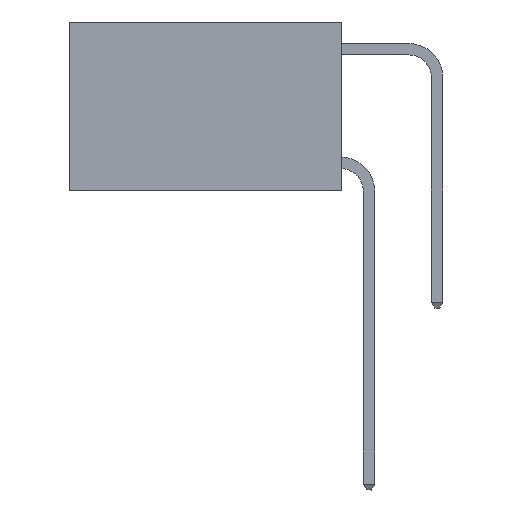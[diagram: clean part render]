
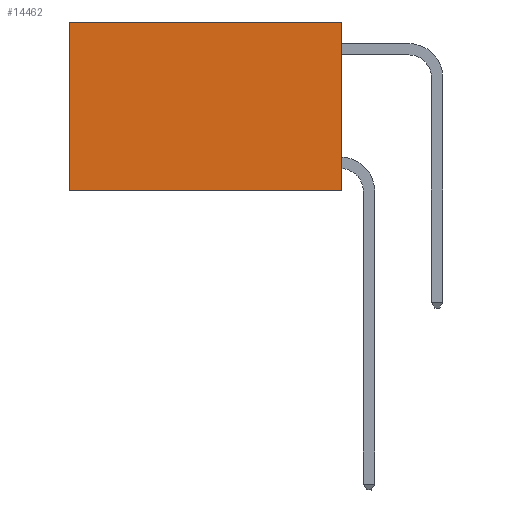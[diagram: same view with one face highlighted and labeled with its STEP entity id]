
A CAD part, left-side view. The second image highlights one B-rep face of the part: STEP entity #14462.
In plain terms, the highlighted planar face has unit normal (-1, 0, 0).
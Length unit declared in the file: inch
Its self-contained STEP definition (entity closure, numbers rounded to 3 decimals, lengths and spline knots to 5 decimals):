
#859 = ORIENTED_EDGE ( 'NONE', *, *, #15998, .F. ) ;
#1146 = LINE ( 'NONE', #4782, #16189 ) ;
#4782 = CARTESIAN_POINT ( 'NONE',  ( 0.2625, 0., 0. ) ) ;
#6386 = VERTEX_POINT ( 'NONE', #22277 ) ;
#6719 = CARTESIAN_POINT ( 'NONE',  ( 0.2625, 0., 0. ) ) ;
#6848 = CARTESIAN_POINT ( 'NONE',  ( 0.2625, 0., -0.37 ) ) ;
#7182 = PLANE ( 'NONE',  #23463 ) ;
#8040 = VECTOR ( 'NONE', #8683, 39.37008 ) ;
#8683 = DIRECTION ( 'NONE',  ( 0., 0., -1. ) ) ;
#8804 = DIRECTION ( 'NONE',  ( 0., 1., 0. ) ) ;
#9157 = DIRECTION ( 'NONE',  ( 0., 0., -1. ) ) ;
#9379 = VECTOR ( 'NONE', #8804, 39.37008 ) ;
#10536 = VECTOR ( 'NONE', #21991, 39.37008 ) ;
#10845 = VERTEX_POINT ( 'NONE', #13858 ) ;
#12106 = FACE_OUTER_BOUND ( 'NONE', #24737, .T. ) ;
#12195 = CARTESIAN_POINT ( 'NONE',  ( 0.2625, 0.6, -0.37 ) ) ;
#13858 = CARTESIAN_POINT ( 'NONE',  ( 0.2625, 0., 0. ) ) ;
#14200 = CARTESIAN_POINT ( 'NONE',  ( 0.2625, 0.6, 0. ) ) ;
#14462 = ADVANCED_FACE ( 'NONE', ( #12106 ), #7182, .F. ) ;
#14595 = LINE ( 'NONE', #6848, #9379 ) ;
#15695 = ORIENTED_EDGE ( 'NONE', *, *, #22775, .T. ) ;
#15878 = EDGE_CURVE ( 'NONE', #24941, #16616, #20851, .T. ) ;
#15998 = EDGE_CURVE ( 'NONE', #10845, #6386, #18435, .T. ) ;
#16189 = VECTOR ( 'NONE', #18462, 39.37008 ) ;
#16616 = VERTEX_POINT ( 'NONE', #12195 ) ;
#16813 = ORIENTED_EDGE ( 'NONE', *, *, #25241, .F. ) ;
#17784 = CARTESIAN_POINT ( 'NONE',  ( 0.2625, 0.6, 0. ) ) ;
#18435 = LINE ( 'NONE', #6719, #8040 ) ;
#18462 = DIRECTION ( 'NONE',  ( 0., 1., 0. ) ) ;
#20814 = DIRECTION ( 'NONE',  ( 1., 0., 0. ) ) ;
#20851 = LINE ( 'NONE', #14200, #10536 ) ;
#21991 = DIRECTION ( 'NONE',  ( 0., 0., -1. ) ) ;
#22277 = CARTESIAN_POINT ( 'NONE',  ( 0.2625, 0., -0.37 ) ) ;
#22719 = CARTESIAN_POINT ( 'NONE',  ( 0.2625, 0., 0. ) ) ;
#22775 = EDGE_CURVE ( 'NONE', #10845, #24941, #1146, .T. ) ;
#23463 = AXIS2_PLACEMENT_3D ( 'NONE', #22719, #20814, #9157 ) ;
#23780 = ORIENTED_EDGE ( 'NONE', *, *, #15878, .T. ) ;
#24737 = EDGE_LOOP ( 'NONE', ( #23780, #16813, #859, #15695 ) ) ;
#24941 = VERTEX_POINT ( 'NONE', #17784 ) ;
#25241 = EDGE_CURVE ( 'NONE', #6386, #16616, #14595, .T. ) ;
